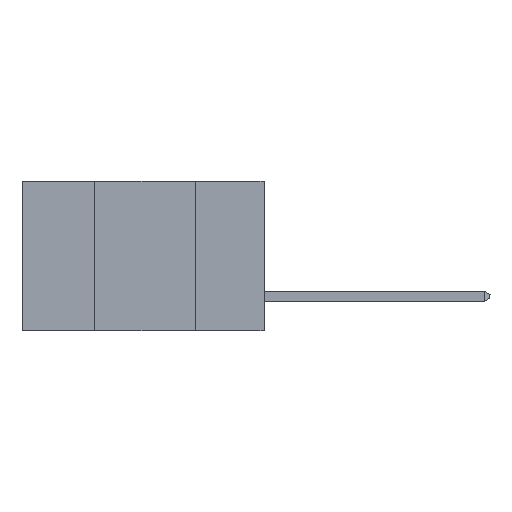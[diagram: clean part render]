
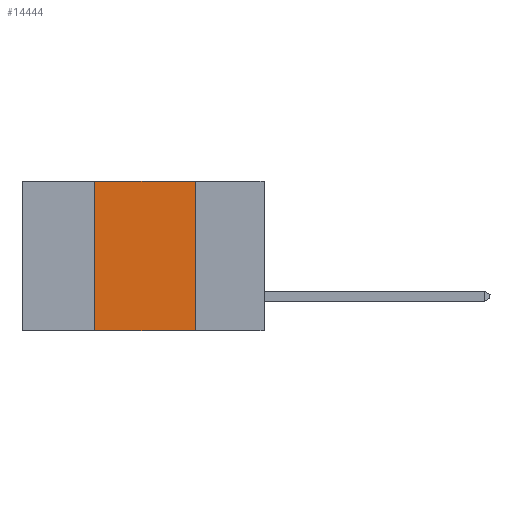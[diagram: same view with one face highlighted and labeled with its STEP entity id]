
A CAD part, left-side view. The second image highlights one B-rep face of the part: STEP entity #14444.
In plain terms, the highlighted planar face has unit normal (-1, 0, 0).
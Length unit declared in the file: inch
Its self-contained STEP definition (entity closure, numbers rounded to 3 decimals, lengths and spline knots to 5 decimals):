
#128 = ORIENTED_EDGE ( 'NONE', *, *, #2874, .F. ) ;
#467 = EDGE_CURVE ( 'NONE', #7721, #712, #1182, .T. ) ;
#481 = DIRECTION ( 'NONE',  ( 0., -1., 0. ) ) ;
#712 = VERTEX_POINT ( 'NONE', #12949 ) ;
#1032 = CARTESIAN_POINT ( 'NONE',  ( 0., 0.42, 0. ) ) ;
#1182 = LINE ( 'NONE', #2928, #13969 ) ;
#1503 = EDGE_LOOP ( 'NONE', ( #15998, #8956, #128, #13581 ) ) ;
#1701 = CARTESIAN_POINT ( 'NONE',  ( 0., 0.6, 0. ) ) ;
#2874 = EDGE_CURVE ( 'NONE', #7721, #14100, #13359, .T. ) ;
#2928 = CARTESIAN_POINT ( 'NONE',  ( 0., 0.6, -0.37 ) ) ;
#2998 = PLANE ( 'NONE',  #7120 ) ;
#3617 = LINE ( 'NONE', #1701, #13106 ) ;
#4564 = EDGE_CURVE ( 'NONE', #6751, #712, #14854, .T. ) ;
#5329 = DIRECTION ( 'NONE',  ( 1., 0., 0. ) ) ;
#5484 = DIRECTION ( 'NONE',  ( 0., 0., -1. ) ) ;
#6751 = VERTEX_POINT ( 'NONE', #14531 ) ;
#7120 = AXIS2_PLACEMENT_3D ( 'NONE', #11470, #5329, #5484 ) ;
#7721 = VERTEX_POINT ( 'NONE', #10954 ) ;
#8956 = ORIENTED_EDGE ( 'NONE', *, *, #12516, .F. ) ;
#10129 = DIRECTION ( 'NONE',  ( 0., 0., -1. ) ) ;
#10547 = FACE_OUTER_BOUND ( 'NONE', #1503, .T. ) ;
#10954 = CARTESIAN_POINT ( 'NONE',  ( 0., 0.42, -0.37 ) ) ;
#11389 = CARTESIAN_POINT ( 'NONE',  ( 0., 0.17, 0. ) ) ;
#11470 = CARTESIAN_POINT ( 'NONE',  ( 0., 0.6, 0. ) ) ;
#11961 = CARTESIAN_POINT ( 'NONE',  ( 0., 0.42, 0. ) ) ;
#12516 = EDGE_CURVE ( 'NONE', #14100, #6751, #3617, .T. ) ;
#12949 = CARTESIAN_POINT ( 'NONE',  ( 0., 0.17, -0.37 ) ) ;
#12967 = VECTOR ( 'NONE', #15815, 39.37008 ) ;
#13106 = VECTOR ( 'NONE', #481, 39.37008 ) ;
#13359 = LINE ( 'NONE', #1032, #12967 ) ;
#13581 = ORIENTED_EDGE ( 'NONE', *, *, #467, .T. ) ;
#13967 = DIRECTION ( 'NONE',  ( 0., -1., 0. ) ) ;
#13969 = VECTOR ( 'NONE', #13967, 39.37008 ) ;
#14100 = VERTEX_POINT ( 'NONE', #11961 ) ;
#14444 = ADVANCED_FACE ( 'NONE', ( #10547 ), #2998, .F. ) ;
#14531 = CARTESIAN_POINT ( 'NONE',  ( 0., 0.17, 0. ) ) ;
#14854 = LINE ( 'NONE', #11389, #16010 ) ;
#15815 = DIRECTION ( 'NONE',  ( 0., 0., 1. ) ) ;
#15998 = ORIENTED_EDGE ( 'NONE', *, *, #4564, .F. ) ;
#16010 = VECTOR ( 'NONE', #10129, 39.37008 ) ;
